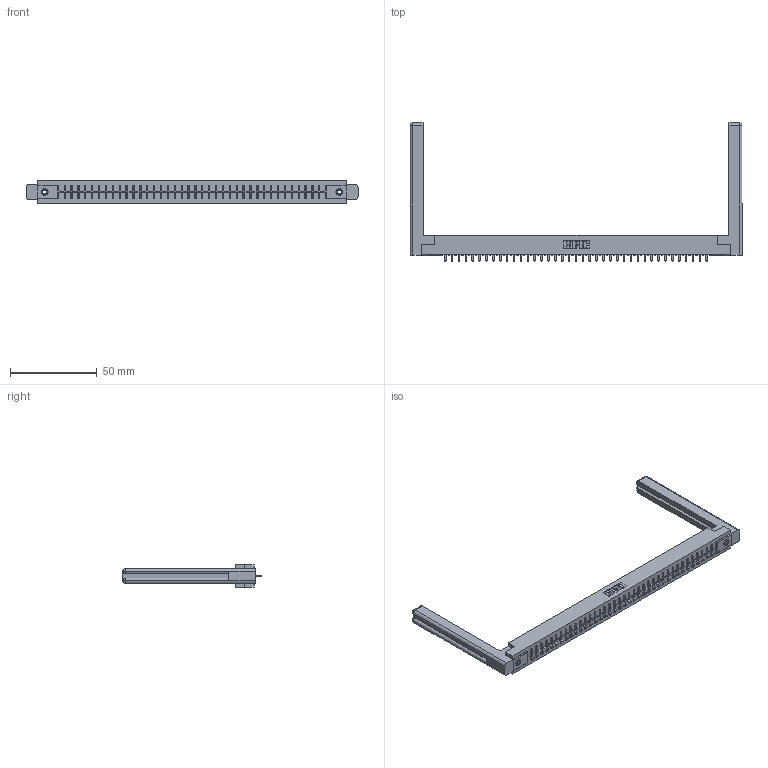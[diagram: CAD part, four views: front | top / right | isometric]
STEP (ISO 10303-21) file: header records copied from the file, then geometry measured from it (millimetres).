
FILE_DESCRIPTION (( 'STEP AP203' ), '1' );
FILE_NAME ('316-039-521-158.STEP', '2018-07-31T05:13:21', ( '' ), ( '' ), 'SwSTEP 2.0', 'SolidWorks 2016', '' );
FILE_SCHEMA (( 'CONFIG_CONTROL_DESIGN' ));
Length unit declared in the file: inch
Products named in the file (5): 306 Part_.156 Dia; 306-290-001_121; 345-250-001_345-250-001-102; 307-220-058; 316-039-521-158
Assembly tree (44 placements, depth 2):
  316-039-521-158
    306 Part_.156 Dia
    306-290-001_121  x39
    345-250-001_345-250-001-102  x2
    307-220-058  x2
Bounding box: 191.16 x 79.53 x 12.7 mm (x, y, z)
Volume: 28141.7 mm3; surface area: 26421.3 mm2
Topology: 44 solids, 44 shells, 2988 faces, 8353 edges, 5346 vertices
Faces by surface type: plane 1985, cylinder 823, sphere 156, cone 12, torus 12
Entity records: 39347 total; most frequent: CARTESIAN_POINT 6615, ORIENTED_EDGE 6500, DIRECTION 6478, EDGE_CURVE 3250, VECTOR 2536, LINE 2536, VERTEX_POINT 2054, AXIS2_PLACEMENT_3D 1971
